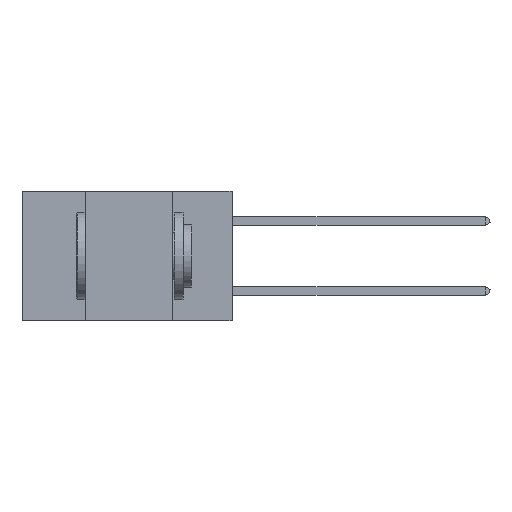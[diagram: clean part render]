
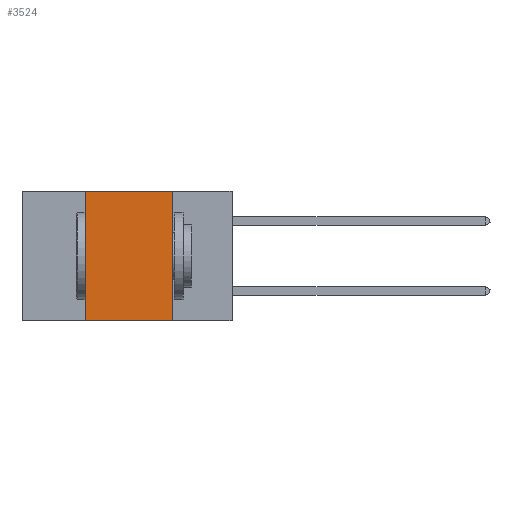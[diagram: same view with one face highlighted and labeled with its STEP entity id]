
A CAD part, left-side view. The second image highlights one B-rep face of the part: STEP entity #3524.
In plain terms, the highlighted planar face has unit normal (-1, 0, 0).
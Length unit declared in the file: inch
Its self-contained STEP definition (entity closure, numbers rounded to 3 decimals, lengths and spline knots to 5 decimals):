
#1012 = FACE_OUTER_BOUND ( 'NONE', #34211, .T. ) ;
#1812 = ORIENTED_EDGE ( 'NONE', *, *, #30633, .F. ) ;
#3493 = EDGE_CURVE ( 'NONE', #13579, #35027, #12652, .T. ) ;
#3524 = ADVANCED_FACE ( 'NONE', ( #1012 ), #41287, .F. ) ;
#5009 = ORIENTED_EDGE ( 'NONE', *, *, #35481, .F. ) ;
#8000 = CARTESIAN_POINT ( 'NONE',  ( 0., 0.17, -0.37 ) ) ;
#8104 = ORIENTED_EDGE ( 'NONE', *, *, #3493, .T. ) ;
#9209 = VECTOR ( 'NONE', #26503, 39.37008 ) ;
#9426 = CARTESIAN_POINT ( 'NONE',  ( 0., 0.42, 0. ) ) ;
#9951 = CARTESIAN_POINT ( 'NONE',  ( 0., 0.17, 0. ) ) ;
#11142 = AXIS2_PLACEMENT_3D ( 'NONE', #18526, #34898, #31700 ) ;
#12320 = VERTEX_POINT ( 'NONE', #18514 ) ;
#12652 = LINE ( 'NONE', #30603, #34712 ) ;
#13579 = VERTEX_POINT ( 'NONE', #14338 ) ;
#13703 = CARTESIAN_POINT ( 'NONE',  ( 0., 0.6, 0. ) ) ;
#14338 = CARTESIAN_POINT ( 'NONE',  ( 0., 0.42, -0.37 ) ) ;
#15917 = VECTOR ( 'NONE', #15930, 39.37008 ) ;
#15930 = DIRECTION ( 'NONE',  ( 0., 0., 1. ) ) ;
#17011 = VECTOR ( 'NONE', #25996, 39.37008 ) ;
#17402 = ORIENTED_EDGE ( 'NONE', *, *, #25943, .F. ) ;
#18514 = CARTESIAN_POINT ( 'NONE',  ( 0., 0.17, 0. ) ) ;
#18526 = CARTESIAN_POINT ( 'NONE',  ( 0., 0.6, 0. ) ) ;
#21265 = LINE ( 'NONE', #13703, #9209 ) ;
#24006 = LINE ( 'NONE', #9951, #17011 ) ;
#24182 = CARTESIAN_POINT ( 'NONE',  ( 0., 0.42, 0. ) ) ;
#25943 = EDGE_CURVE ( 'NONE', #40043, #12320, #21265, .T. ) ;
#25996 = DIRECTION ( 'NONE',  ( 0., 0., -1. ) ) ;
#26503 = DIRECTION ( 'NONE',  ( 0., -1., 0. ) ) ;
#30603 = CARTESIAN_POINT ( 'NONE',  ( 0., 0.6, -0.37 ) ) ;
#30633 = EDGE_CURVE ( 'NONE', #13579, #40043, #34959, .T. ) ;
#31700 = DIRECTION ( 'NONE',  ( 0., 0., -1. ) ) ;
#33815 = DIRECTION ( 'NONE',  ( 0., -1., 0. ) ) ;
#34211 = EDGE_LOOP ( 'NONE', ( #5009, #17402, #1812, #8104 ) ) ;
#34712 = VECTOR ( 'NONE', #33815, 39.37008 ) ;
#34898 = DIRECTION ( 'NONE',  ( 1., 0., 0. ) ) ;
#34959 = LINE ( 'NONE', #9426, #15917 ) ;
#35027 = VERTEX_POINT ( 'NONE', #8000 ) ;
#35481 = EDGE_CURVE ( 'NONE', #12320, #35027, #24006, .T. ) ;
#40043 = VERTEX_POINT ( 'NONE', #24182 ) ;
#41287 = PLANE ( 'NONE',  #11142 ) ;
